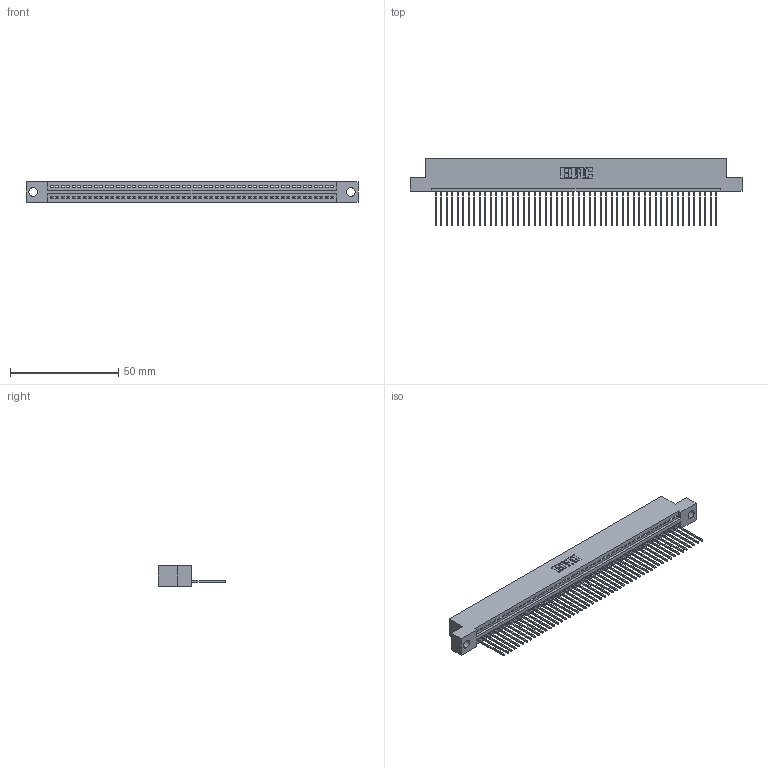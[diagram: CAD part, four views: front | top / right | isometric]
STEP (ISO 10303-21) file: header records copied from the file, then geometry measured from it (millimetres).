
FILE_DESCRIPTION (( 'STEP AP203' ), '1' );
FILE_NAME ('345-052-542-104.STEP', '2021-05-28T15:27:14', ( '' ), ( '' ), 'SwSTEP 2.0', 'SolidWorks 2020', '' );
FILE_SCHEMA (( 'CONFIG_CONTROL_DESIGN' ));
Length unit declared in the file: inch
Products named in the file (3): 345 Part_Flush Mounting Lugs - 0.156 Dia-TI; 345-292-001_345-293-142; 345-052-542-104
Assembly tree (53 placements, depth 2):
  345-052-542-104
    345 Part_Flush Mounting Lugs - 0.156 Dia-TI
    345-292-001_345-293-142  x52
Bounding box: 153.29 x 31.29 x 9.4 mm (x, y, z)
Volume: 14651.2 mm3; surface area: 20180.2 mm2
Topology: 53 solids, 53 shells, 3156 faces, 9529 edges, 6282 vertices
Faces by surface type: plane 2174, cylinder 982
Entity records: 38227 total; most frequent: CARTESIAN_POINT 6630, ORIENTED_EDGE 6614, DIRECTION 5775, EDGE_CURVE 3307, LINE 2967, VECTOR 2967, VERTEX_POINT 2202, AXIS2_PLACEMENT_3D 1404
